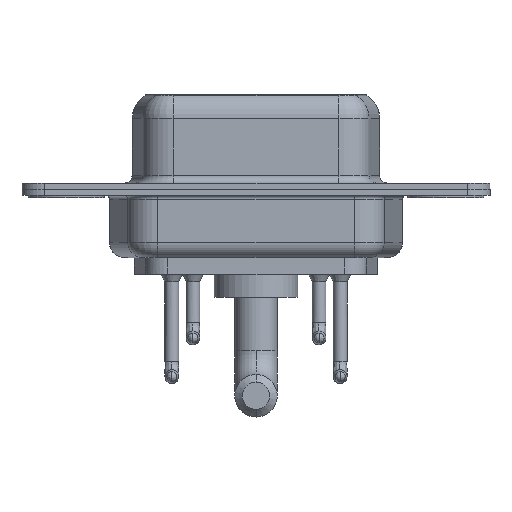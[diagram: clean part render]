
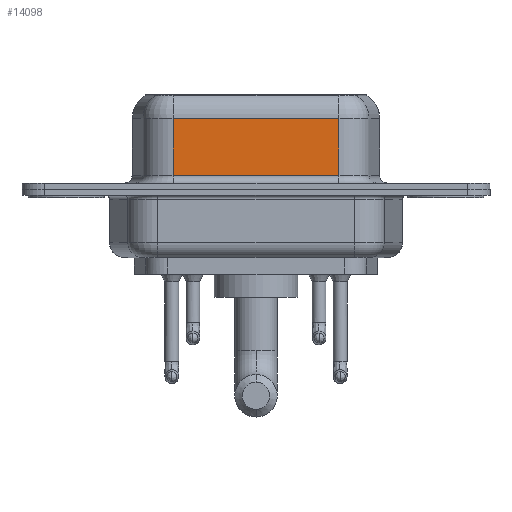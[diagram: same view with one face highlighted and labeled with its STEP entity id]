
A CAD part, front view. The second image highlights one B-rep face of the part: STEP entity #14098.
In plain terms, the highlighted planar face has unit normal (0, -1, 0).
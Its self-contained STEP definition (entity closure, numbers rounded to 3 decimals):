
#109 = AXIS2_PLACEMENT_3D ( 'NONE', #4293, #1946, #12093 ) ;
#182 = EDGE_CURVE ( 'NONE', #1528, #13588, #8813, .T. ) ;
#1267 = VECTOR ( 'NONE', #14505, 1000. ) ;
#1395 = CARTESIAN_POINT ( 'NONE',  ( 17.962, -3.95, 6.4 ) ) ;
#1454 = FACE_OUTER_BOUND ( 'NONE', #2295, .T. ) ;
#1466 = CARTESIAN_POINT ( 'NONE',  ( 7.038, -3.95, 0.9 ) ) ;
#1528 = VERTEX_POINT ( 'NONE', #7721 ) ;
#1617 = VERTEX_POINT ( 'NONE', #5729 ) ;
#1740 = VECTOR ( 'NONE', #10338, 1000. ) ;
#1946 = DIRECTION ( 'NONE',  ( 0., 1., 0. ) ) ;
#2295 = EDGE_LOOP ( 'NONE', ( #9332, #6389, #10366, #5773 ) ) ;
#2413 = LINE ( 'NONE', #1395, #1740 ) ;
#2621 = PLANE ( 'NONE',  #109 ) ;
#3240 = CARTESIAN_POINT ( 'NONE',  ( 7.038, -3.95, 6.4 ) ) ;
#3242 = CARTESIAN_POINT ( 'NONE',  ( 17.962, -3.95, 4.65 ) ) ;
#3291 = EDGE_CURVE ( 'NONE', #13588, #1617, #10020, .T. ) ;
#3315 = DIRECTION ( 'NONE',  ( -1., 0., 0. ) ) ;
#4180 = VECTOR ( 'NONE', #3315, 1000. ) ;
#4199 = LINE ( 'NONE', #3242, #4180 ) ;
#4293 = CARTESIAN_POINT ( 'NONE',  ( 17.962, -3.95, 6.4 ) ) ;
#5660 = CARTESIAN_POINT ( 'NONE',  ( 17.962, -3.95, 4.65 ) ) ;
#5729 = CARTESIAN_POINT ( 'NONE',  ( 17.962, -3.95, 0.9 ) ) ;
#5773 = ORIENTED_EDGE ( 'NONE', *, *, #3291, .T. ) ;
#6389 = ORIENTED_EDGE ( 'NONE', *, *, #6929, .T. ) ;
#6929 = EDGE_CURVE ( 'NONE', #11346, #1528, #4199, .T. ) ;
#7601 = VECTOR ( 'NONE', #11013, 1000. ) ;
#7721 = CARTESIAN_POINT ( 'NONE',  ( 7.038, -3.95, 4.65 ) ) ;
#8813 = LINE ( 'NONE', #3240, #7601 ) ;
#9332 = ORIENTED_EDGE ( 'NONE', *, *, #13522, .F. ) ;
#10020 = LINE ( 'NONE', #13406, #1267 ) ;
#10338 = DIRECTION ( 'NONE',  ( 0., 0., -1. ) ) ;
#10366 = ORIENTED_EDGE ( 'NONE', *, *, #182, .T. ) ;
#11013 = DIRECTION ( 'NONE',  ( 0., 0., -1. ) ) ;
#11346 = VERTEX_POINT ( 'NONE', #5660 ) ;
#12093 = DIRECTION ( 'NONE',  ( -1., 0., 0. ) ) ;
#13406 = CARTESIAN_POINT ( 'NONE',  ( 17.962, -3.95, 0.9 ) ) ;
#13522 = EDGE_CURVE ( 'NONE', #11346, #1617, #2413, .T. ) ;
#13588 = VERTEX_POINT ( 'NONE', #1466 ) ;
#14098 = ADVANCED_FACE ( 'NONE', ( #1454 ), #2621, .F. ) ;
#14505 = DIRECTION ( 'NONE',  ( 1., 0., 0. ) ) ;
